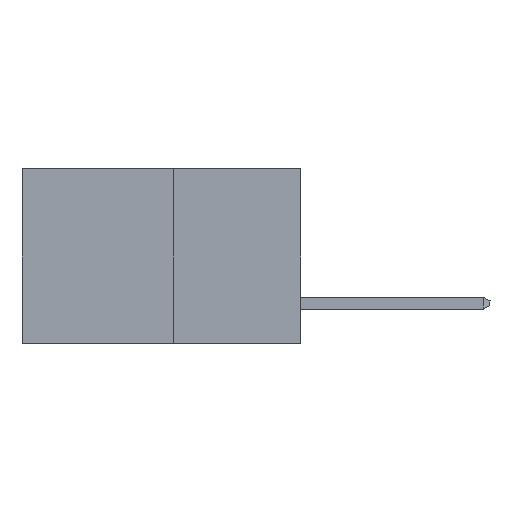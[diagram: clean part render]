
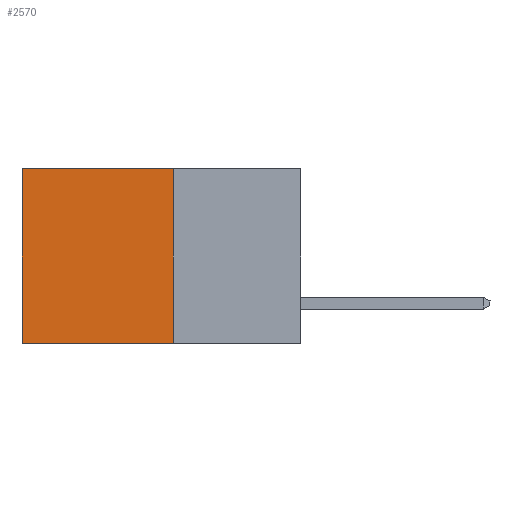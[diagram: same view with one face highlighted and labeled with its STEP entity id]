
A CAD part, left-side view. The second image highlights one B-rep face of the part: STEP entity #2570.
In plain terms, the highlighted planar face has unit normal (-1, 0, 0).
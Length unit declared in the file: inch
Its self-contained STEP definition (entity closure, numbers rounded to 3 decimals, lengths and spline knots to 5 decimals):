
#61 = VECTOR ( 'NONE', #6504, 39.37008 ) ;
#179 = DIRECTION ( 'NONE',  ( 1., 0., 0. ) ) ;
#196 = DIRECTION ( 'NONE',  ( 0., 1., 0. ) ) ;
#572 = EDGE_CURVE ( 'NONE', #5243, #1225, #2651, .T. ) ;
#893 = ORIENTED_EDGE ( 'NONE', *, *, #3266, .F. ) ;
#1225 = VERTEX_POINT ( 'NONE', #2767 ) ;
#1356 = VECTOR ( 'NONE', #2683, 39.37008 ) ;
#2230 = EDGE_LOOP ( 'NONE', ( #3715, #893, #8963, #9473 ) ) ;
#2357 = EDGE_CURVE ( 'NONE', #5243, #3013, #3636, .T. ) ;
#2570 = ADVANCED_FACE ( 'NONE', ( #5630 ), #6547, .F. ) ;
#2651 = LINE ( 'NONE', #5534, #61 ) ;
#2683 = DIRECTION ( 'NONE',  ( 0., 0., -1. ) ) ;
#2767 = CARTESIAN_POINT ( 'NONE',  ( 0.277, 0.59, 0. ) ) ;
#2872 = VECTOR ( 'NONE', #196, 39.37008 ) ;
#3013 = VERTEX_POINT ( 'NONE', #10436 ) ;
#3170 = LINE ( 'NONE', #6247, #2872 ) ;
#3264 = CARTESIAN_POINT ( 'NONE',  ( 0.277, 0.59, -0.37 ) ) ;
#3266 = EDGE_CURVE ( 'NONE', #3013, #4723, #3170, .T. ) ;
#3554 = CARTESIAN_POINT ( 'NONE',  ( 0.277, 0.27, 0. ) ) ;
#3636 = LINE ( 'NONE', #9715, #5769 ) ;
#3715 = ORIENTED_EDGE ( 'NONE', *, *, #4057, .T. ) ;
#4057 = EDGE_CURVE ( 'NONE', #1225, #4723, #8282, .T. ) ;
#4474 = CARTESIAN_POINT ( 'NONE',  ( 0.277, 0.27, -0.37 ) ) ;
#4595 = DIRECTION ( 'NONE',  ( 0., 0., -1. ) ) ;
#4723 = VERTEX_POINT ( 'NONE', #7161 ) ;
#5243 = VERTEX_POINT ( 'NONE', #3554 ) ;
#5534 = CARTESIAN_POINT ( 'NONE',  ( 0.277, 0.27, 0. ) ) ;
#5630 = FACE_OUTER_BOUND ( 'NONE', #2230, .T. ) ;
#5769 = VECTOR ( 'NONE', #9163, 39.37008 ) ;
#6247 = CARTESIAN_POINT ( 'NONE',  ( 0.277, 0.27, -0.37 ) ) ;
#6497 = AXIS2_PLACEMENT_3D ( 'NONE', #4474, #179, #4595 ) ;
#6504 = DIRECTION ( 'NONE',  ( 0., 1., 0. ) ) ;
#6547 = PLANE ( 'NONE',  #6497 ) ;
#7161 = CARTESIAN_POINT ( 'NONE',  ( 0.277, 0.59, -0.37 ) ) ;
#8282 = LINE ( 'NONE', #3264, #1356 ) ;
#8963 = ORIENTED_EDGE ( 'NONE', *, *, #2357, .F. ) ;
#9163 = DIRECTION ( 'NONE',  ( 0., 0., -1. ) ) ;
#9473 = ORIENTED_EDGE ( 'NONE', *, *, #572, .T. ) ;
#9715 = CARTESIAN_POINT ( 'NONE',  ( 0.277, 0.27, -0.37 ) ) ;
#10436 = CARTESIAN_POINT ( 'NONE',  ( 0.277, 0.27, -0.37 ) ) ;
